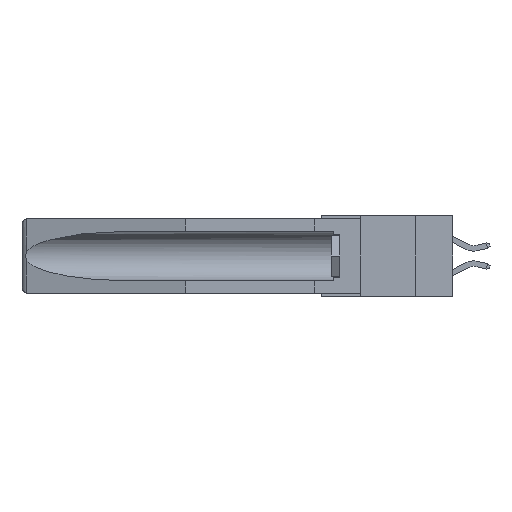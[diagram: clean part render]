
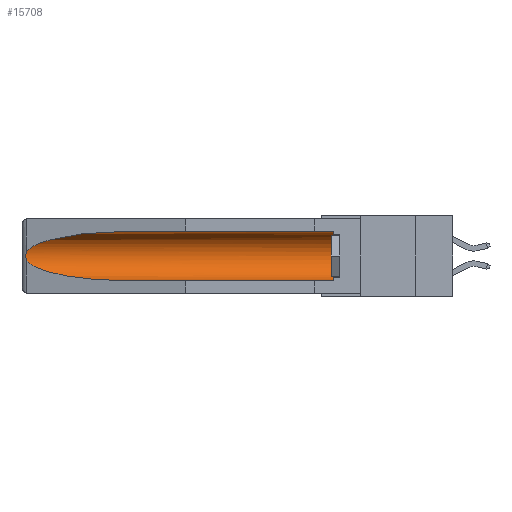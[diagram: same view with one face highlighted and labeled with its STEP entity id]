
A CAD part, left-side view. The second image highlights one B-rep face of the part: STEP entity #15708.
In plain terms, the highlighted cylindrical face has radius 2.857 mm (diameter 5.715 mm), a partial arc.
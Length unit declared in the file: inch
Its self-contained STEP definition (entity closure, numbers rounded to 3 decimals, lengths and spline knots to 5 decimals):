
#27 = VERTEX_POINT ( 'NONE', #9206 ) ;
#125 = CARTESIAN_POINT ( 'NONE',  ( 0.21114, 1.30732, -0.059 ) ) ;
#444 = EDGE_LOOP ( 'NONE', ( #14444, #2210, #8760, #13231, #9800, #1497 ) ) ;
#824 = DIRECTION ( 'NONE',  ( 0., -1., 0. ) ) ;
#1044 = AXIS2_PLACEMENT_3D ( 'NONE', #16007, #824, #2235 ) ;
#1497 = ORIENTED_EDGE ( 'NONE', *, *, #4940, .T. ) ;
#1874 = CARTESIAN_POINT ( 'NONE',  ( 0.2673, 1.5327, -0.16383 ) ) ;
#1911 =( BOUNDED_CURVE ( )  B_SPLINE_CURVE ( 3, ( #14205, #125, #2990, #7280 ),
 .UNSPECIFIED., .F., .T. ) 
 B_SPLINE_CURVE_WITH_KNOTS ( ( 4, 4 ),
 ( 4.71239, 6.08839 ),
 .UNSPECIFIED. ) 
 CURVE ( )  GEOMETRIC_REPRESENTATION_ITEM ( )  RATIONAL_B_SPLINE_CURVE ( ( 1., 0.848, 0.848, 1. ) ) 
 REPRESENTATION_ITEM ( '' )  );
#2210 = ORIENTED_EDGE ( 'NONE', *, *, #5007, .T. ) ;
#2235 = DIRECTION ( 'NONE',  ( 0., 0., 1. ) ) ;
#2838 = DIRECTION ( 'NONE',  ( 0., 1., 0. ) ) ;
#2990 = CARTESIAN_POINT ( 'NONE',  ( 0.25451, 1.48313, -0.09465 ) ) ;
#3220 = CARTESIAN_POINT ( 'NONE',  ( 0.26654, 1.53092, -0.15636 ) ) ;
#3323 = VERTEX_POINT ( 'NONE', #15272 ) ;
#3410 = CARTESIAN_POINT ( 'NONE',  ( 0.2673, 1.53269, -0.17917 ) ) ;
#4081 = VERTEX_POINT ( 'NONE', #9602 ) ;
#4367 = VERTEX_POINT ( 'NONE', #8395 ) ;
#4545 = CARTESIAN_POINT ( 'NONE',  ( 0.26597, 1.5296, -0.19026 ) ) ;
#4673 = DIRECTION ( 'NONE',  ( 0., 1., 0. ) ) ;
#4674 = CARTESIAN_POINT ( 'NONE',  ( 0.26655, 1.53094, -0.18657 ) ) ;
#4940 = EDGE_CURVE ( 'NONE', #27, #3323, #6658, .T. ) ;
#5007 = EDGE_CURVE ( 'NONE', #4367, #13598, #6699, .T. ) ;
#5046 = CARTESIAN_POINT ( 'NONE',  ( 0.26537, 1.52718, -0.19328 ) ) ;
#5341 = CARTESIAN_POINT ( 'NONE',  ( 0.21114, 1.30732, -0.284 ) ) ;
#6239 = CARTESIAN_POINT ( 'NONE',  ( 0.155, 0.126, -0.284 ) ) ;
#6330 = CARTESIAN_POINT ( 'NONE',  ( 0.26537, 1.52718, -0.19328 ) ) ;
#6658 = LINE ( 'NONE', #7196, #10942 ) ;
#6699 = B_SPLINE_CURVE_WITH_KNOTS ( 'NONE', 3,
 ( #16934, #8730, #3220, #1874, #12795, #8600, #3410, #4674, #4545, #14124 ),
 .UNSPECIFIED., .F., .F.,
 ( 4, 2, 2, 2, 4 ),
 ( 0., 0.00029, 0.00058, 0.00087, 0.00117 ),
 .UNSPECIFIED. ) ;
#6735 = FACE_OUTER_BOUND ( 'NONE', #444, .T. ) ;
#7196 = CARTESIAN_POINT ( 'NONE',  ( 0.155, -0.30754, -0.059 ) ) ;
#7280 = CARTESIAN_POINT ( 'NONE',  ( 0.26537, 1.52718, -0.14972 ) ) ;
#7794 = LINE ( 'NONE', #17245, #15369 ) ;
#8395 = CARTESIAN_POINT ( 'NONE',  ( 0.26537, 1.52718, -0.14972 ) ) ;
#8600 = CARTESIAN_POINT ( 'NONE',  ( 0.2675, 1.53308, -0.17534 ) ) ;
#8730 = CARTESIAN_POINT ( 'NONE',  ( 0.26597, 1.52961, -0.15275 ) ) ;
#8760 = ORIENTED_EDGE ( 'NONE', *, *, #9649, .T. ) ;
#8964 = DIRECTION ( 'NONE',  ( 0., 0., 1. ) ) ;
#9206 = CARTESIAN_POINT ( 'NONE',  ( 0.155, 0.126, -0.059 ) ) ;
#9475 = AXIS2_PLACEMENT_3D ( 'NONE', #14478, #4673, #8964 ) ;
#9602 = CARTESIAN_POINT ( 'NONE',  ( 0.155, 1.07973, -0.284 ) ) ;
#9649 = EDGE_CURVE ( 'NONE', #13598, #4081, #13633, .T. ) ;
#9800 = ORIENTED_EDGE ( 'NONE', *, *, #15307, .T. ) ;
#10606 = CYLINDRICAL_SURFACE ( 'NONE', #9475, 0.1125 ) ;
#10942 = VECTOR ( 'NONE', #2838, 39.37008 ) ;
#12795 = CARTESIAN_POINT ( 'NONE',  ( 0.2675, 1.53308, -0.16763 ) ) ;
#13008 = CIRCLE ( 'NONE', #1044, 0.1125 ) ;
#13231 = ORIENTED_EDGE ( 'NONE', *, *, #15778, .F. ) ;
#13598 = VERTEX_POINT ( 'NONE', #6330 ) ;
#13633 =( BOUNDED_CURVE ( )  B_SPLINE_CURVE ( 3, ( #5046, #14681, #5341, #16275 ),
 .UNSPECIFIED., .F., .T. ) 
 B_SPLINE_CURVE_WITH_KNOTS ( ( 4, 4 ),
 ( 0.1948, 1.5708 ),
 .UNSPECIFIED. ) 
 CURVE ( )  GEOMETRIC_REPRESENTATION_ITEM ( )  RATIONAL_B_SPLINE_CURVE ( ( 1., 0.848, 0.848, 1. ) ) 
 REPRESENTATION_ITEM ( '' )  );
#14124 = CARTESIAN_POINT ( 'NONE',  ( 0.26537, 1.52718, -0.19328 ) ) ;
#14205 = CARTESIAN_POINT ( 'NONE',  ( 0.155, 1.07973, -0.059 ) ) ;
#14444 = ORIENTED_EDGE ( 'NONE', *, *, #15140, .T. ) ;
#14478 = CARTESIAN_POINT ( 'NONE',  ( 0.155, -0.30754, -0.1715 ) ) ;
#14681 = CARTESIAN_POINT ( 'NONE',  ( 0.25451, 1.48313, -0.24835 ) ) ;
#14940 = VERTEX_POINT ( 'NONE', #6239 ) ;
#15140 = EDGE_CURVE ( 'NONE', #3323, #4367, #1911, .T. ) ;
#15272 = CARTESIAN_POINT ( 'NONE',  ( 0.155, 1.07973, -0.059 ) ) ;
#15307 = EDGE_CURVE ( 'NONE', #14940, #27, #13008, .T. ) ;
#15369 = VECTOR ( 'NONE', #17111, 39.37008 ) ;
#15708 = ADVANCED_FACE ( 'NONE', ( #6735 ), #10606, .F. ) ;
#15778 = EDGE_CURVE ( 'NONE', #14940, #4081, #7794, .T. ) ;
#16007 = CARTESIAN_POINT ( 'NONE',  ( 0.155, 0.126, -0.1715 ) ) ;
#16275 = CARTESIAN_POINT ( 'NONE',  ( 0.155, 1.07973, -0.284 ) ) ;
#16934 = CARTESIAN_POINT ( 'NONE',  ( 0.26537, 1.52718, -0.14972 ) ) ;
#17111 = DIRECTION ( 'NONE',  ( 0., 1., 0. ) ) ;
#17245 = CARTESIAN_POINT ( 'NONE',  ( 0.155, -0.30754, -0.284 ) ) ;
